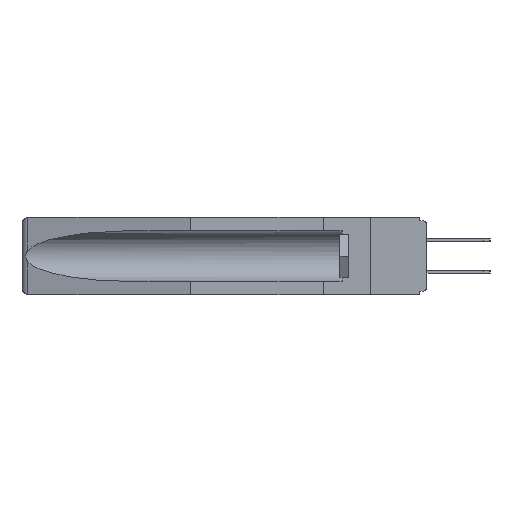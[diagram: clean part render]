
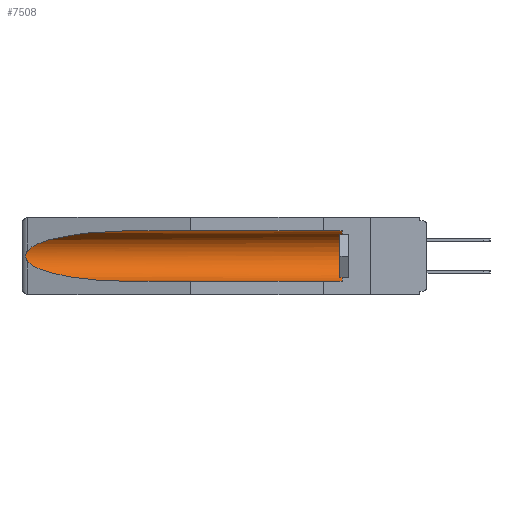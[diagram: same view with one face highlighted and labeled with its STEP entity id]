
A CAD part, left-side view. The second image highlights one B-rep face of the part: STEP entity #7508.
In plain terms, the highlighted cylindrical face has radius 2.857 mm (diameter 5.715 mm), a partial arc.
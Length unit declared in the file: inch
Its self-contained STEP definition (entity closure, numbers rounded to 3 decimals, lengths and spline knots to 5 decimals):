
#9 = LINE ( 'NONE', #14554, #7735 ) ;
#756 = CARTESIAN_POINT ( 'NONE',  ( 0.26597, 1.5296, -0.19026 ) ) ;
#2357 = CARTESIAN_POINT ( 'NONE',  ( 0.155, 0.126, -0.1715 ) ) ;
#2788 = AXIS2_PLACEMENT_3D ( 'NONE', #12157, #24923, #18677 ) ;
#3005 = VERTEX_POINT ( 'NONE', #17520 ) ;
#3827 = CARTESIAN_POINT ( 'NONE',  ( 0.26537, 1.52718, -0.19328 ) ) ;
#4228 = VERTEX_POINT ( 'NONE', #3827 ) ;
#4311 = DIRECTION ( 'NONE',  ( 0., 1., 0. ) ) ;
#5309 = CARTESIAN_POINT ( 'NONE',  ( 0.155, 1.07973, -0.284 ) ) ;
#5838 = ORIENTED_EDGE ( 'NONE', *, *, #24284, .T. ) ;
#6522 = CARTESIAN_POINT ( 'NONE',  ( 0.2673, 1.5327, -0.16383 ) ) ;
#6541 =( BOUNDED_CURVE ( )  B_SPLINE_CURVE ( 3, ( #12081, #14264, #26798, #13972 ),
 .UNSPECIFIED., .F., .F. ) 
 B_SPLINE_CURVE_WITH_KNOTS ( ( 4, 4 ),
 ( 4.71239, 6.08839 ),
 .UNSPECIFIED. ) 
 CURVE ( )  GEOMETRIC_REPRESENTATION_ITEM ( )  RATIONAL_B_SPLINE_CURVE ( ( 1., 0.848, 0.848, 1. ) ) 
 REPRESENTATION_ITEM ( '' )  );
#6649 = CARTESIAN_POINT ( 'NONE',  ( 0.155, 1.07973, -0.059 ) ) ;
#7248 = CARTESIAN_POINT ( 'NONE',  ( 0.26537, 1.52718, -0.19328 ) ) ;
#7326 = VERTEX_POINT ( 'NONE', #19125 ) ;
#7478 = CARTESIAN_POINT ( 'NONE',  ( 0.21114, 1.30732, -0.284 ) ) ;
#7508 = ADVANCED_FACE ( 'NONE', ( #20052 ), #27380, .F. ) ;
#7735 = VECTOR ( 'NONE', #25511, 39.37008 ) ;
#7746 = CARTESIAN_POINT ( 'NONE',  ( 0.25451, 1.48313, -0.24835 ) ) ;
#9052 = EDGE_CURVE ( 'NONE', #4228, #23774, #11801, .T. ) ;
#9212 = CARTESIAN_POINT ( 'NONE',  ( 0.2675, 1.53308, -0.17534 ) ) ;
#9303 = CARTESIAN_POINT ( 'NONE',  ( 0.26654, 1.53092, -0.15636 ) ) ;
#9705 = ORIENTED_EDGE ( 'NONE', *, *, #13439, .T. ) ;
#9876 = CARTESIAN_POINT ( 'NONE',  ( 0.26537, 1.52718, -0.19328 ) ) ;
#10875 = DIRECTION ( 'NONE',  ( 0., 0., 1. ) ) ;
#11369 = CARTESIAN_POINT ( 'NONE',  ( 0.155, 1.07973, -0.284 ) ) ;
#11801 =( BOUNDED_CURVE ( )  B_SPLINE_CURVE ( 3, ( #9876, #7746, #7478, #5309 ),
 .UNSPECIFIED., .F., .F. ) 
 B_SPLINE_CURVE_WITH_KNOTS ( ( 4, 4 ),
 ( 0.1948, 1.5708 ),
 .UNSPECIFIED. ) 
 CURVE ( )  GEOMETRIC_REPRESENTATION_ITEM ( )  RATIONAL_B_SPLINE_CURVE ( ( 1., 0.848, 0.848, 1. ) ) 
 REPRESENTATION_ITEM ( '' )  );
#12081 = CARTESIAN_POINT ( 'NONE',  ( 0.155, 1.07973, -0.059 ) ) ;
#12157 = CARTESIAN_POINT ( 'NONE',  ( 0.155, -0.30754, -0.1715 ) ) ;
#12407 = EDGE_CURVE ( 'NONE', #13478, #3005, #6541, .T. ) ;
#12798 = CARTESIAN_POINT ( 'NONE',  ( 0.155, -0.30754, -0.059 ) ) ;
#13439 = EDGE_CURVE ( 'NONE', #7326, #13478, #23762, .T. ) ;
#13478 = VERTEX_POINT ( 'NONE', #6649 ) ;
#13596 = CARTESIAN_POINT ( 'NONE',  ( 0.26655, 1.53094, -0.18657 ) ) ;
#13689 = CARTESIAN_POINT ( 'NONE',  ( 0.2675, 1.53308, -0.16763 ) ) ;
#13972 = CARTESIAN_POINT ( 'NONE',  ( 0.26537, 1.52718, -0.14972 ) ) ;
#14264 = CARTESIAN_POINT ( 'NONE',  ( 0.21114, 1.30732, -0.059 ) ) ;
#14554 = CARTESIAN_POINT ( 'NONE',  ( 0.155, -0.30754, -0.284 ) ) ;
#15610 = CARTESIAN_POINT ( 'NONE',  ( 0.26537, 1.52718, -0.14972 ) ) ;
#16010 = EDGE_CURVE ( 'NONE', #18888, #23774, #9, .T. ) ;
#16115 = CARTESIAN_POINT ( 'NONE',  ( 0.155, 0.126, -0.284 ) ) ;
#17520 = CARTESIAN_POINT ( 'NONE',  ( 0.26537, 1.52718, -0.14972 ) ) ;
#17916 = ORIENTED_EDGE ( 'NONE', *, *, #21226, .T. ) ;
#18677 = DIRECTION ( 'NONE',  ( 0., 0., 1. ) ) ;
#18888 = VERTEX_POINT ( 'NONE', #16115 ) ;
#19125 = CARTESIAN_POINT ( 'NONE',  ( 0.155, 0.126, -0.059 ) ) ;
#19820 = ORIENTED_EDGE ( 'NONE', *, *, #9052, .T. ) ;
#20052 = FACE_OUTER_BOUND ( 'NONE', #25213, .T. ) ;
#21226 = EDGE_CURVE ( 'NONE', #18888, #7326, #25324, .T. ) ;
#21949 = CARTESIAN_POINT ( 'NONE',  ( 0.26597, 1.52961, -0.15275 ) ) ;
#22285 = B_SPLINE_CURVE_WITH_KNOTS ( 'NONE', 3,
 ( #15610, #21949, #9303, #6522, #13689, #9212, #24360, #13596, #756, #7248 ),
 .UNSPECIFIED., .F., .F.,
 ( 4, 2, 2, 2, 4 ),
 ( 0., 0.00029, 0.00058, 0.00087, 0.00117 ),
 .UNSPECIFIED. ) ;
#23114 = AXIS2_PLACEMENT_3D ( 'NONE', #2357, #23705, #10875 ) ;
#23705 = DIRECTION ( 'NONE',  ( 0., -1., 0. ) ) ;
#23762 = LINE ( 'NONE', #12798, #25762 ) ;
#23774 = VERTEX_POINT ( 'NONE', #11369 ) ;
#24115 = ORIENTED_EDGE ( 'NONE', *, *, #12407, .T. ) ;
#24284 = EDGE_CURVE ( 'NONE', #3005, #4228, #22285, .T. ) ;
#24360 = CARTESIAN_POINT ( 'NONE',  ( 0.2673, 1.53269, -0.17917 ) ) ;
#24923 = DIRECTION ( 'NONE',  ( 0., 1., 0. ) ) ;
#24961 = ORIENTED_EDGE ( 'NONE', *, *, #16010, .F. ) ;
#25213 = EDGE_LOOP ( 'NONE', ( #24115, #5838, #19820, #24961, #17916, #9705 ) ) ;
#25324 = CIRCLE ( 'NONE', #23114, 0.1125 ) ;
#25511 = DIRECTION ( 'NONE',  ( 0., 1., 0. ) ) ;
#25762 = VECTOR ( 'NONE', #4311, 39.37008 ) ;
#26798 = CARTESIAN_POINT ( 'NONE',  ( 0.25451, 1.48313, -0.09465 ) ) ;
#27380 = CYLINDRICAL_SURFACE ( 'NONE', #2788, 0.1125 ) ;
